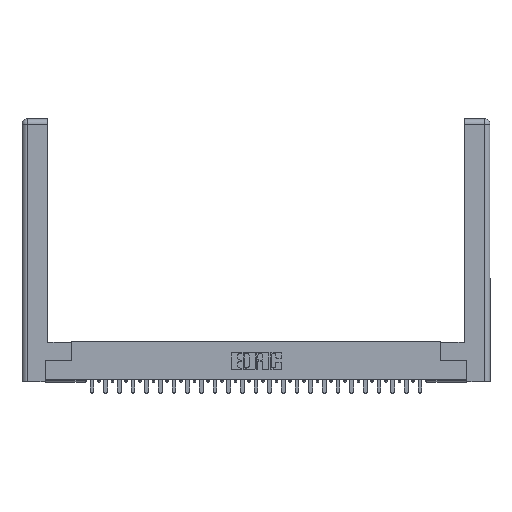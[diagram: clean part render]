
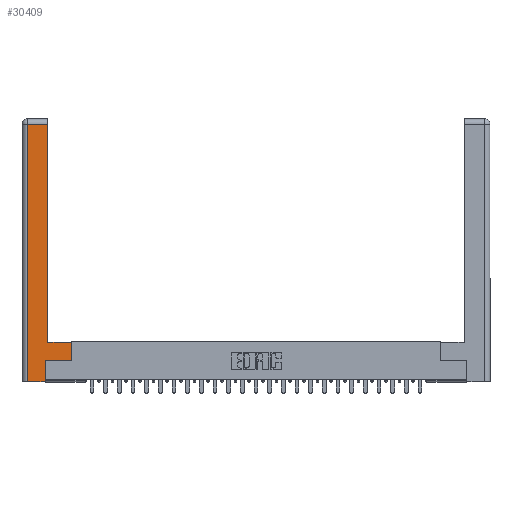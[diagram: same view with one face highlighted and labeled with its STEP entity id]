
A CAD part, top view. The second image highlights one B-rep face of the part: STEP entity #30409.
In plain terms, the highlighted planar face has unit normal (0, 0, 1).
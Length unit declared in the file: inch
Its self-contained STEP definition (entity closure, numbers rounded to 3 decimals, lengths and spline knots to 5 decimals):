
#41 = LINE ( 'NONE', #18939, #5440 ) ;
#307 = VERTEX_POINT ( 'NONE', #20629 ) ;
#650 = VECTOR ( 'NONE', #20288, 39.37008 ) ;
#693 = VECTOR ( 'NONE', #15892, 39.37008 ) ;
#820 = VERTEX_POINT ( 'NONE', #5675 ) ;
#1051 = LINE ( 'NONE', #19999, #15959 ) ;
#1335 = ORIENTED_EDGE ( 'NONE', *, *, #28065, .T. ) ;
#2141 = CARTESIAN_POINT ( 'NONE',  ( 0.295, 0.45, 0. ) ) ;
#2222 = CARTESIAN_POINT ( 'NONE',  ( 0.565, 0.245, 0. ) ) ;
#2316 = EDGE_CURVE ( 'NONE', #25087, #8508, #1051, .T. ) ;
#2584 = DIRECTION ( 'NONE',  ( -1., 0., 0. ) ) ;
#3595 = DIRECTION ( 'NONE',  ( 0., 1., 0. ) ) ;
#3634 = EDGE_CURVE ( 'NONE', #820, #12230, #18583, .T. ) ;
#3935 = ORIENTED_EDGE ( 'NONE', *, *, #15940, .T. ) ;
#4554 = DIRECTION ( 'NONE',  ( 1., 0., 0. ) ) ;
#4564 = LINE ( 'NONE', #27552, #693 ) ;
#5096 = VERTEX_POINT ( 'NONE', #18660 ) ;
#5184 = DIRECTION ( 'NONE',  ( -1., 0., 0. ) ) ;
#5440 = VECTOR ( 'NONE', #26129, 39.37008 ) ;
#5675 = CARTESIAN_POINT ( 'NONE',  ( 0.265, 0., 0. ) ) ;
#7673 = ORIENTED_EDGE ( 'NONE', *, *, #3634, .T. ) ;
#8044 = CARTESIAN_POINT ( 'NONE',  ( 0.265, 0., 0. ) ) ;
#8508 = VERTEX_POINT ( 'NONE', #2141 ) ;
#8866 = EDGE_CURVE ( 'NONE', #14700, #307, #4564, .T. ) ;
#9972 = ORIENTED_EDGE ( 'NONE', *, *, #21199, .T. ) ;
#10008 = CARTESIAN_POINT ( 'NONE',  ( 0.0615, 0., 0. ) ) ;
#12230 = VERTEX_POINT ( 'NONE', #30224 ) ;
#12575 = LINE ( 'NONE', #28048, #24014 ) ;
#13080 = EDGE_CURVE ( 'NONE', #8508, #14700, #41, .T. ) ;
#13279 = EDGE_CURVE ( 'NONE', #307, #5096, #18375, .T. ) ;
#13822 = ORIENTED_EDGE ( 'NONE', *, *, #13080, .T. ) ;
#14095 = VECTOR ( 'NONE', #4554, 39.37008 ) ;
#14700 = VERTEX_POINT ( 'NONE', #20721 ) ;
#14837 = DIRECTION ( 'NONE',  ( 0., 1., 0. ) ) ;
#15136 = AXIS2_PLACEMENT_3D ( 'NONE', #19779, #24997, #2584 ) ;
#15407 = EDGE_LOOP ( 'NONE', ( #13822, #26366, #22278, #1335, #7673, #3935, #9972, #22877 ) ) ;
#15892 = DIRECTION ( 'NONE',  ( -1., 0., 0. ) ) ;
#15940 = EDGE_CURVE ( 'NONE', #12230, #20947, #26741, .T. ) ;
#15959 = VECTOR ( 'NONE', #5184, 39.37008 ) ;
#18375 = LINE ( 'NONE', #10008, #20670 ) ;
#18583 = LINE ( 'NONE', #29263, #19745 ) ;
#18660 = CARTESIAN_POINT ( 'NONE',  ( 0.0615, 0., 0. ) ) ;
#18939 = CARTESIAN_POINT ( 'NONE',  ( 0.295, 3., 0. ) ) ;
#19745 = VECTOR ( 'NONE', #14837, 39.37008 ) ;
#19779 = CARTESIAN_POINT ( 'NONE',  ( 0., 0., 0. ) ) ;
#19999 = CARTESIAN_POINT ( 'NONE',  ( 0.295, 0.45, 0. ) ) ;
#20288 = DIRECTION ( 'NONE',  ( 1., 0., 0. ) ) ;
#20629 = CARTESIAN_POINT ( 'NONE',  ( 0.0615, 2.94, 0. ) ) ;
#20670 = VECTOR ( 'NONE', #27282, 39.37008 ) ;
#20721 = CARTESIAN_POINT ( 'NONE',  ( 0.295, 2.94, 0. ) ) ;
#20947 = VERTEX_POINT ( 'NONE', #2222 ) ;
#21199 = EDGE_CURVE ( 'NONE', #20947, #25087, #12575, .T. ) ;
#22278 = ORIENTED_EDGE ( 'NONE', *, *, #13279, .T. ) ;
#22540 = PLANE ( 'NONE',  #15136 ) ;
#22877 = ORIENTED_EDGE ( 'NONE', *, *, #2316, .T. ) ;
#23647 = CARTESIAN_POINT ( 'NONE',  ( 0.565, 0.245, 0. ) ) ;
#24014 = VECTOR ( 'NONE', #3595, 39.37008 ) ;
#24997 = DIRECTION ( 'NONE',  ( 0., 0., -1. ) ) ;
#25087 = VERTEX_POINT ( 'NONE', #27587 ) ;
#26129 = DIRECTION ( 'NONE',  ( 0., 1., 0. ) ) ;
#26366 = ORIENTED_EDGE ( 'NONE', *, *, #8866, .T. ) ;
#26416 = FACE_OUTER_BOUND ( 'NONE', #15407, .T. ) ;
#26741 = LINE ( 'NONE', #23647, #14095 ) ;
#27282 = DIRECTION ( 'NONE',  ( 0., -1., 0. ) ) ;
#27434 = LINE ( 'NONE', #8044, #650 ) ;
#27552 = CARTESIAN_POINT ( 'NONE',  ( 0.0615, 2.94, 0. ) ) ;
#27587 = CARTESIAN_POINT ( 'NONE',  ( 0.565, 0.45, 0. ) ) ;
#28048 = CARTESIAN_POINT ( 'NONE',  ( 0.565, 0.45, 0. ) ) ;
#28065 = EDGE_CURVE ( 'NONE', #5096, #820, #27434, .T. ) ;
#29263 = CARTESIAN_POINT ( 'NONE',  ( 0.265, 0.245, 0. ) ) ;
#30224 = CARTESIAN_POINT ( 'NONE',  ( 0.265, 0.245, 0. ) ) ;
#30409 = ADVANCED_FACE ( 'NONE', ( #26416 ), #22540, .F. ) ;
